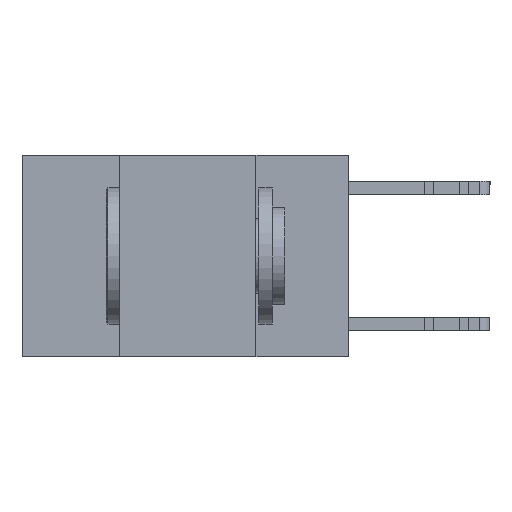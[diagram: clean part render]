
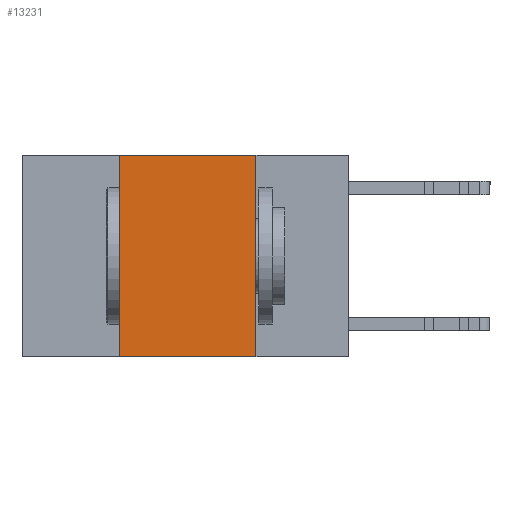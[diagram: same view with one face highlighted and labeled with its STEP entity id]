
A CAD part, left-side view. The second image highlights one B-rep face of the part: STEP entity #13231.
In plain terms, the highlighted planar face has unit normal (-1, 0, 0).
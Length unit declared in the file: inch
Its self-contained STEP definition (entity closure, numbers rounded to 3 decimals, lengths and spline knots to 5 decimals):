
#1513 = ORIENTED_EDGE ( 'NONE', *, *, #7413, .T. ) ;
#2271 = VECTOR ( 'NONE', #10402, 39.37008 ) ;
#2887 = LINE ( 'NONE', #12036, #10151 ) ;
#4029 = PLANE ( 'NONE',  #16008 ) ;
#4086 = DIRECTION ( 'NONE',  ( 0., 0., 1. ) ) ;
#4577 = VERTEX_POINT ( 'NONE', #28731 ) ;
#5974 = FACE_OUTER_BOUND ( 'NONE', #17267, .T. ) ;
#6227 = CARTESIAN_POINT ( 'NONE',  ( 0., 0.6, -0.37 ) ) ;
#6662 = CARTESIAN_POINT ( 'NONE',  ( 0., 0.42, -0.37 ) ) ;
#7283 = VECTOR ( 'NONE', #4086, 39.37008 ) ;
#7413 = EDGE_CURVE ( 'NONE', #9528, #4577, #24248, .T. ) ;
#9528 = VERTEX_POINT ( 'NONE', #6662 ) ;
#9733 = EDGE_CURVE ( 'NONE', #25461, #4577, #2887, .T. ) ;
#10151 = VECTOR ( 'NONE', #16988, 39.37008 ) ;
#10402 = DIRECTION ( 'NONE',  ( 0., -1., 0. ) ) ;
#12036 = CARTESIAN_POINT ( 'NONE',  ( 0., 0.17, 0. ) ) ;
#13231 = ADVANCED_FACE ( 'NONE', ( #5974 ), #4029, .F. ) ;
#15293 = DIRECTION ( 'NONE',  ( 0., -1., 0. ) ) ;
#15936 = EDGE_CURVE ( 'NONE', #23746, #25461, #23332, .T. ) ;
#16008 = AXIS2_PLACEMENT_3D ( 'NONE', #17978, #22504, #22645 ) ;
#16988 = DIRECTION ( 'NONE',  ( 0., 0., -1. ) ) ;
#17267 = EDGE_LOOP ( 'NONE', ( #28096, #26088, #21412, #1513 ) ) ;
#17882 = LINE ( 'NONE', #26933, #7283 ) ;
#17978 = CARTESIAN_POINT ( 'NONE',  ( 0., 0.6, 0. ) ) ;
#19480 = VECTOR ( 'NONE', #15293, 39.37008 ) ;
#19691 = CARTESIAN_POINT ( 'NONE',  ( 0., 0.17, 0. ) ) ;
#21412 = ORIENTED_EDGE ( 'NONE', *, *, #27989, .F. ) ;
#22283 = CARTESIAN_POINT ( 'NONE',  ( 0., 0.42, 0. ) ) ;
#22504 = DIRECTION ( 'NONE',  ( 1., 0., 0. ) ) ;
#22645 = DIRECTION ( 'NONE',  ( 0., 0., -1. ) ) ;
#23332 = LINE ( 'NONE', #29144, #19480 ) ;
#23746 = VERTEX_POINT ( 'NONE', #22283 ) ;
#24248 = LINE ( 'NONE', #6227, #2271 ) ;
#25461 = VERTEX_POINT ( 'NONE', #19691 ) ;
#26088 = ORIENTED_EDGE ( 'NONE', *, *, #15936, .F. ) ;
#26933 = CARTESIAN_POINT ( 'NONE',  ( 0., 0.42, 0. ) ) ;
#27989 = EDGE_CURVE ( 'NONE', #9528, #23746, #17882, .T. ) ;
#28096 = ORIENTED_EDGE ( 'NONE', *, *, #9733, .F. ) ;
#28731 = CARTESIAN_POINT ( 'NONE',  ( 0., 0.17, -0.37 ) ) ;
#29144 = CARTESIAN_POINT ( 'NONE',  ( 0., 0.6, 0. ) ) ;
